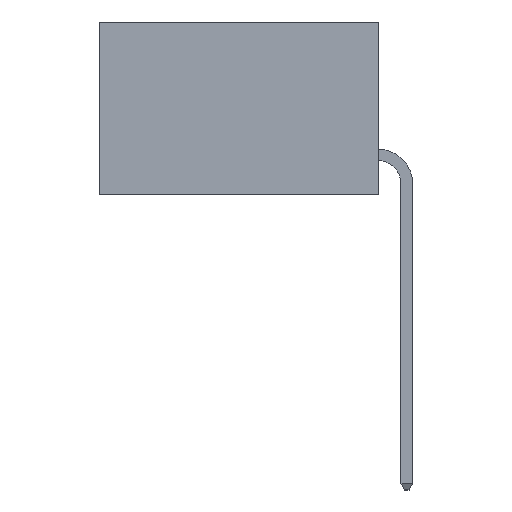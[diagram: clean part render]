
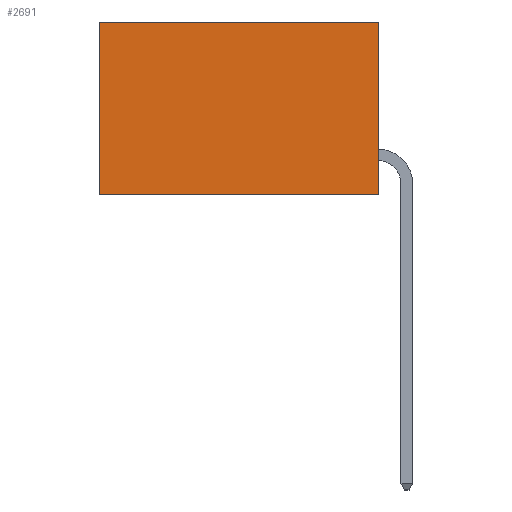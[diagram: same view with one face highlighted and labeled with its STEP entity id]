
A CAD part, left-side view. The second image highlights one B-rep face of the part: STEP entity #2691.
In plain terms, the highlighted planar face has unit normal (-1, 0, 0).
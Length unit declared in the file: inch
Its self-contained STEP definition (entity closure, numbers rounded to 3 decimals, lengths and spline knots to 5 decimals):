
#30 = CARTESIAN_POINT ( 'NONE',  ( 0.2615, 0.6, -0.37 ) ) ;
#144 = VECTOR ( 'NONE', #4347, 39.37008 ) ;
#459 = DIRECTION ( 'NONE',  ( 0., 0., -1. ) ) ;
#1237 = LINE ( 'NONE', #30, #9425 ) ;
#2019 = ORIENTED_EDGE ( 'NONE', *, *, #5712, .T. ) ;
#2034 = CARTESIAN_POINT ( 'NONE',  ( 0.2615, 0., -0.37 ) ) ;
#2044 = ORIENTED_EDGE ( 'NONE', *, *, #7118, .F. ) ;
#2143 = ORIENTED_EDGE ( 'NONE', *, *, #7555, .F. ) ;
#2259 = DIRECTION ( 'NONE',  ( 0., 1., 0. ) ) ;
#2285 = ORIENTED_EDGE ( 'NONE', *, *, #6173, .T. ) ;
#2290 = CARTESIAN_POINT ( 'NONE',  ( 0.2615, 0., -0.37 ) ) ;
#2691 = ADVANCED_FACE ( 'NONE', ( #8349 ), #5831, .F. ) ;
#3143 = DIRECTION ( 'NONE',  ( 0., 1., 0. ) ) ;
#4086 = CARTESIAN_POINT ( 'NONE',  ( 0.2615, 0., 0. ) ) ;
#4347 = DIRECTION ( 'NONE',  ( 0., 0., -1. ) ) ;
#4612 = CARTESIAN_POINT ( 'NONE',  ( 0.2615, 0.6, -0.37 ) ) ;
#5712 = EDGE_CURVE ( 'NONE', #6024, #7803, #1237, .T. ) ;
#5748 = DIRECTION ( 'NONE',  ( 0., 0., -1. ) ) ;
#5750 = DIRECTION ( 'NONE',  ( 1., 0., 0. ) ) ;
#5762 = CARTESIAN_POINT ( 'NONE',  ( 0.2615, 0., -0.37 ) ) ;
#5831 = PLANE ( 'NONE',  #10059 ) ;
#5847 = CARTESIAN_POINT ( 'NONE',  ( 0.2615, 0., 0. ) ) ;
#6024 = VERTEX_POINT ( 'NONE', #9369 ) ;
#6173 = EDGE_CURVE ( 'NONE', #9344, #6024, #9827, .T. ) ;
#7118 = EDGE_CURVE ( 'NONE', #9767, #7803, #7950, .T. ) ;
#7308 = EDGE_LOOP ( 'NONE', ( #2019, #2044, #2143, #2285 ) ) ;
#7555 = EDGE_CURVE ( 'NONE', #9344, #9767, #8990, .T. ) ;
#7803 = VERTEX_POINT ( 'NONE', #4612 ) ;
#7950 = LINE ( 'NONE', #2290, #8401 ) ;
#8349 = FACE_OUTER_BOUND ( 'NONE', #7308, .T. ) ;
#8401 = VECTOR ( 'NONE', #2259, 39.37008 ) ;
#8990 = LINE ( 'NONE', #2034, #144 ) ;
#9256 = CARTESIAN_POINT ( 'NONE',  ( 0.2615, 0., -0.37 ) ) ;
#9344 = VERTEX_POINT ( 'NONE', #5847 ) ;
#9369 = CARTESIAN_POINT ( 'NONE',  ( 0.2615, 0.6, 0. ) ) ;
#9425 = VECTOR ( 'NONE', #459, 39.37008 ) ;
#9629 = VECTOR ( 'NONE', #3143, 39.37008 ) ;
#9767 = VERTEX_POINT ( 'NONE', #9256 ) ;
#9827 = LINE ( 'NONE', #4086, #9629 ) ;
#10059 = AXIS2_PLACEMENT_3D ( 'NONE', #5762, #5750, #5748 ) ;
